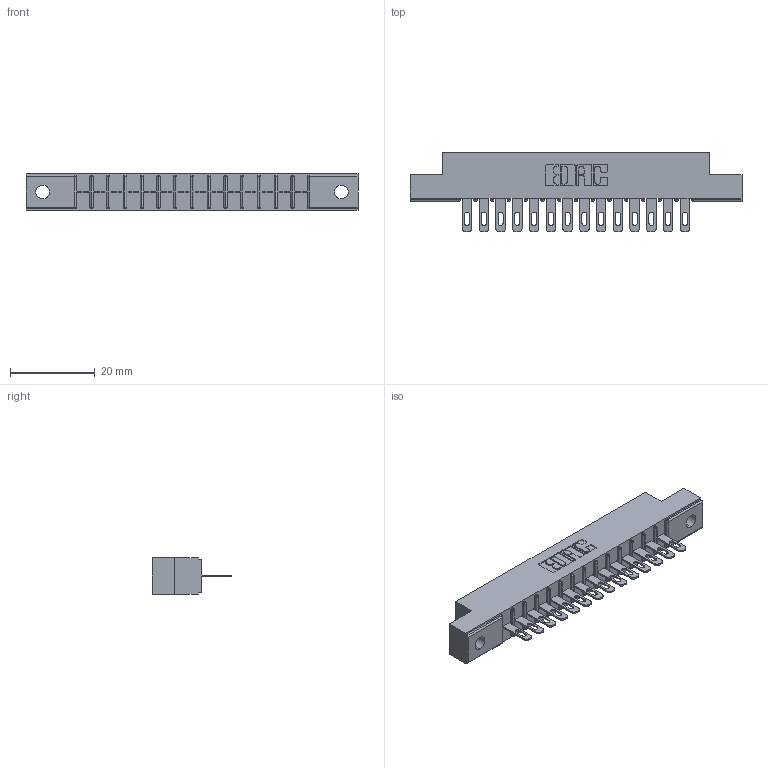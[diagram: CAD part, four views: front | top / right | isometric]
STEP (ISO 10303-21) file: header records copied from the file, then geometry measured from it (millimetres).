
FILE_DESCRIPTION (( 'STEP AP203' ), '1' );
FILE_NAME ('356-014-500-102.STEP', '2018-08-01T19:02:16', ( '' ), ( '' ), 'SwSTEP 2.0', 'SolidWorks 2016', '' );
FILE_SCHEMA (( 'CONFIG_CONTROL_DESIGN' ));
Length unit declared in the file: inch
Products named in the file (3): 306 Part_.128 Dia; 306-290-001_100; 356-014-500-102
Assembly tree (15 placements, depth 2):
  356-014-500-102
    306 Part_.128 Dia
    306-290-001_100  x14
Bounding box: 78.49 x 18.87 x 8.71 mm (x, y, z)
Volume: 5336.9 mm3; surface area: 7609.3 mm2
Topology: 15 solids, 15 shells, 1180 faces, 3326 edges, 2140 vertices
Faces by surface type: plane 768, cylinder 356, sphere 56
Entity records: 16849 total; most frequent: CARTESIAN_POINT 2825, ORIENTED_EDGE 2796, DIRECTION 2790, EDGE_CURVE 1398, VECTOR 1076, LINE 1076, VERTEX_POINT 892, AXIS2_PLACEMENT_3D 857
